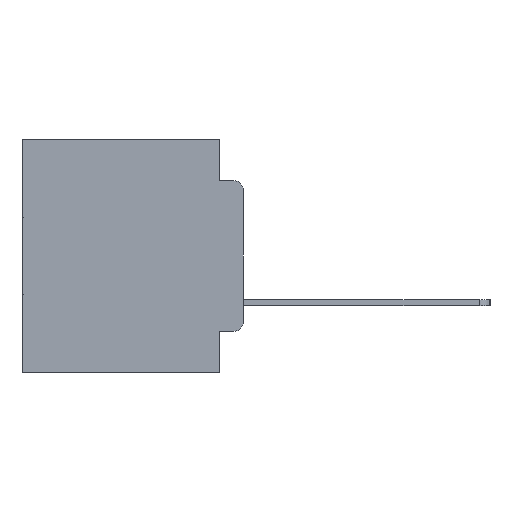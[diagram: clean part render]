
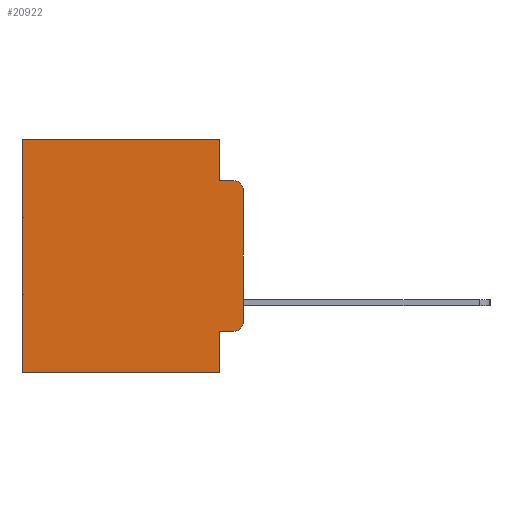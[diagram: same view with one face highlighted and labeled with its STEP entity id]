
A CAD part, left-side view. The second image highlights one B-rep face of the part: STEP entity #20922.
In plain terms, the highlighted planar face has unit normal (-1, 0, 0).
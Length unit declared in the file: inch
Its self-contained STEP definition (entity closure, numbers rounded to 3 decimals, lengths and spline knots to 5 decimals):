
#493 = AXIS2_PLACEMENT_3D ( 'NONE', #9079, #25450, #11430 ) ;
#741 = DIRECTION ( 'NONE',  ( 0., 0., -1. ) ) ;
#940 = EDGE_CURVE ( 'NONE', #2656, #14650, #9458, .T. ) ;
#990 = ORIENTED_EDGE ( 'NONE', *, *, #26136, .F. ) ;
#1664 = CARTESIAN_POINT ( 'NONE',  ( 0.298, 0.051, 0. ) ) ;
#2491 = VECTOR ( 'NONE', #12191, 39.37008 ) ;
#2656 = VERTEX_POINT ( 'NONE', #13262 ) ;
#2822 = VECTOR ( 'NONE', #24871, 39.37008 ) ;
#3473 = DIRECTION ( 'NONE',  ( -1., 0., 0. ) ) ;
#4259 = VECTOR ( 'NONE', #16731, 39.37008 ) ;
#4405 = ORIENTED_EDGE ( 'NONE', *, *, #27386, .T. ) ;
#4605 = DIRECTION ( 'NONE',  ( 0., -1., 0. ) ) ;
#5601 = VERTEX_POINT ( 'NONE', #24631 ) ;
#5667 = CIRCLE ( 'NONE', #493, 0.02 ) ;
#5853 = FACE_OUTER_BOUND ( 'NONE', #21934, .T. ) ;
#6124 = CARTESIAN_POINT ( 'NONE',  ( 0.298, 0., -0.3915 ) ) ;
#7294 = VERTEX_POINT ( 'NONE', #19104 ) ;
#7591 = LINE ( 'NONE', #23215, #25529 ) ;
#8105 = CARTESIAN_POINT ( 'NONE',  ( 0.298, 0.051, 0. ) ) ;
#9044 = LINE ( 'NONE', #22520, #2822 ) ;
#9079 = CARTESIAN_POINT ( 'NONE',  ( 0.298, 0.02, -0.3915 ) ) ;
#9218 = EDGE_CURVE ( 'NONE', #21249, #7294, #9044, .T. ) ;
#9458 = LINE ( 'NONE', #21658, #2491 ) ;
#10315 = LINE ( 'NONE', #1664, #22749 ) ;
#10421 = VERTEX_POINT ( 'NONE', #25000 ) ;
#10465 = LINE ( 'NONE', #26026, #4259 ) ;
#10654 = LINE ( 'NONE', #13097, #22376 ) ;
#10682 = EDGE_CURVE ( 'NONE', #5601, #10421, #10465, .T. ) ;
#11281 = EDGE_CURVE ( 'NONE', #21749, #21249, #18476, .T. ) ;
#11430 = DIRECTION ( 'NONE',  ( 0., 0., -1. ) ) ;
#12191 = DIRECTION ( 'NONE',  ( 0., 0., -1. ) ) ;
#12443 = PLANE ( 'NONE',  #20219 ) ;
#12753 = CARTESIAN_POINT ( 'NONE',  ( 0.298, 0.02, -0.4115 ) ) ;
#13097 = CARTESIAN_POINT ( 'NONE',  ( 0.298, 0.473, 0. ) ) ;
#13262 = CARTESIAN_POINT ( 'NONE',  ( 0.298, 0., -0.1085 ) ) ;
#13462 = CARTESIAN_POINT ( 'NONE',  ( 0.298, 0.051, -0.5 ) ) ;
#14650 = VERTEX_POINT ( 'NONE', #6124 ) ;
#14822 = DIRECTION ( 'NONE',  ( 1., 0., 0. ) ) ;
#14898 = VERTEX_POINT ( 'NONE', #21032 ) ;
#15827 = LINE ( 'NONE', #19329, #27517 ) ;
#16731 = DIRECTION ( 'NONE',  ( 0., -1., 0. ) ) ;
#17415 = DIRECTION ( 'NONE',  ( 0., 0., -1. ) ) ;
#17488 = CARTESIAN_POINT ( 'NONE',  ( 0.298, 0.02, -0.1085 ) ) ;
#17625 = ORIENTED_EDGE ( 'NONE', *, *, #29837, .T. ) ;
#17783 = DIRECTION ( 'NONE',  ( 0., 0., -1. ) ) ;
#17810 = CARTESIAN_POINT ( 'NONE',  ( 0.298, 0.051, -0.4115 ) ) ;
#17864 = CIRCLE ( 'NONE', #29241, 0.02 ) ;
#18222 = ORIENTED_EDGE ( 'NONE', *, *, #10682, .F. ) ;
#18476 = LINE ( 'NONE', #19754, #23978 ) ;
#19104 = CARTESIAN_POINT ( 'NONE',  ( 0.298, 0.473, -0.5 ) ) ;
#19329 = CARTESIAN_POINT ( 'NONE',  ( 0.298, 0., 0. ) ) ;
#19692 = ORIENTED_EDGE ( 'NONE', *, *, #940, .F. ) ;
#19754 = CARTESIAN_POINT ( 'NONE',  ( 0.298, 0.051, 0. ) ) ;
#19834 = DIRECTION ( 'NONE',  ( 0., 0., -1. ) ) ;
#20070 = ORIENTED_EDGE ( 'NONE', *, *, #11281, .F. ) ;
#20219 = AXIS2_PLACEMENT_3D ( 'NONE', #26447, #14822, #741 ) ;
#20561 = ORIENTED_EDGE ( 'NONE', *, *, #9218, .F. ) ;
#20922 = ADVANCED_FACE ( 'NONE', ( #5853 ), #12443, .F. ) ;
#21032 = CARTESIAN_POINT ( 'NONE',  ( 0.298, 0.473, 0. ) ) ;
#21249 = VERTEX_POINT ( 'NONE', #13462 ) ;
#21276 = ORIENTED_EDGE ( 'NONE', *, *, #30046, .T. ) ;
#21658 = CARTESIAN_POINT ( 'NONE',  ( 0.298, 0., 0. ) ) ;
#21749 = VERTEX_POINT ( 'NONE', #17810 ) ;
#21934 = EDGE_LOOP ( 'NONE', ( #19692, #26651, #18222, #990, #17625, #21276, #20561, #20070, #28136, #4405 ) ) ;
#21965 = EDGE_CURVE ( 'NONE', #21749, #23312, #7591, .T. ) ;
#22376 = VECTOR ( 'NONE', #17783, 39.37008 ) ;
#22520 = CARTESIAN_POINT ( 'NONE',  ( 0.298, 0., -0.5 ) ) ;
#22707 = EDGE_CURVE ( 'NONE', #2656, #10421, #17864, .T. ) ;
#22749 = VECTOR ( 'NONE', #25102, 39.37008 ) ;
#23215 = CARTESIAN_POINT ( 'NONE',  ( 0.298, 0.051, -0.4115 ) ) ;
#23312 = VERTEX_POINT ( 'NONE', #12753 ) ;
#23978 = VECTOR ( 'NONE', #17415, 39.37008 ) ;
#24042 = DIRECTION ( 'NONE',  ( 0., 1., 0. ) ) ;
#24631 = CARTESIAN_POINT ( 'NONE',  ( 0.298, 0.051, -0.0885 ) ) ;
#24871 = DIRECTION ( 'NONE',  ( 0., 1., 0. ) ) ;
#25000 = CARTESIAN_POINT ( 'NONE',  ( 0.298, 0.02, -0.0885 ) ) ;
#25102 = DIRECTION ( 'NONE',  ( 0., 0., -1. ) ) ;
#25450 = DIRECTION ( 'NONE',  ( -1., 0., 0. ) ) ;
#25529 = VECTOR ( 'NONE', #4605, 39.37008 ) ;
#26026 = CARTESIAN_POINT ( 'NONE',  ( 0.298, 0.051, -0.0885 ) ) ;
#26136 = EDGE_CURVE ( 'NONE', #29353, #5601, #10315, .T. ) ;
#26447 = CARTESIAN_POINT ( 'NONE',  ( 0.298, 0., 0. ) ) ;
#26651 = ORIENTED_EDGE ( 'NONE', *, *, #22707, .T. ) ;
#27386 = EDGE_CURVE ( 'NONE', #23312, #14650, #5667, .T. ) ;
#27517 = VECTOR ( 'NONE', #24042, 39.37008 ) ;
#28136 = ORIENTED_EDGE ( 'NONE', *, *, #21965, .T. ) ;
#29241 = AXIS2_PLACEMENT_3D ( 'NONE', #17488, #3473, #19834 ) ;
#29353 = VERTEX_POINT ( 'NONE', #8105 ) ;
#29837 = EDGE_CURVE ( 'NONE', #29353, #14898, #15827, .T. ) ;
#30046 = EDGE_CURVE ( 'NONE', #14898, #7294, #10654, .T. ) ;
